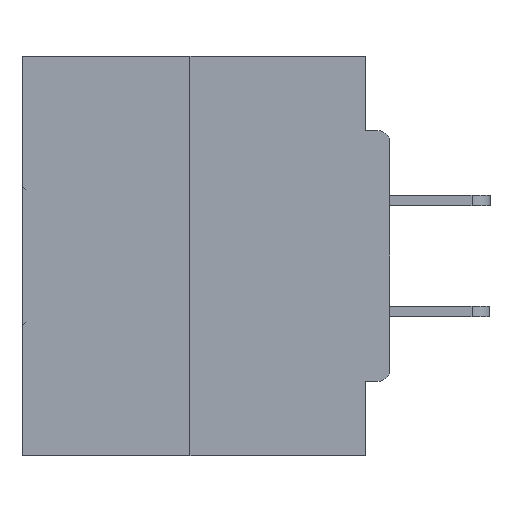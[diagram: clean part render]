
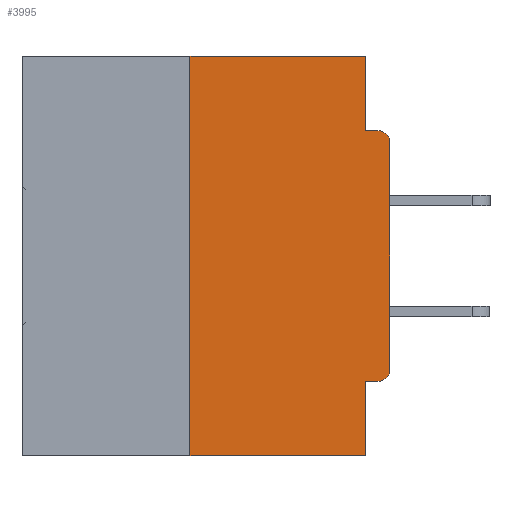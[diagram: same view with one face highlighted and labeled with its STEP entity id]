
A CAD part, left-side view. The second image highlights one B-rep face of the part: STEP entity #3995.
In plain terms, the highlighted planar face has unit normal (-1, 0, 0).
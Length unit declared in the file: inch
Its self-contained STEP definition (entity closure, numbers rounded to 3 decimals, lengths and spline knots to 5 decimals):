
#2 = CARTESIAN_POINT ( 'NONE',  ( 0., 0., -0.0935 ) ) ;
#969 = VERTEX_POINT ( 'NONE', #18899 ) ;
#1359 = CARTESIAN_POINT ( 'NONE',  ( 0., 0., -0.4065 ) ) ;
#1875 = ORIENTED_EDGE ( 'NONE', *, *, #18897, .F. ) ;
#2118 = AXIS2_PLACEMENT_3D ( 'NONE', #34022, #30119, #33000 ) ;
#2420 = EDGE_LOOP ( 'NONE', ( #34603, #5709, #41791, #29876, #35113, #34415, #11903, #22578, #1875, #41406 ) ) ;
#2688 = DIRECTION ( 'NONE',  ( 0., -1., 0. ) ) ;
#3995 = ADVANCED_FACE ( 'NONE', ( #31853 ), #4235, .F. ) ;
#4235 = PLANE ( 'NONE',  #2118 ) ;
#5149 = CARTESIAN_POINT ( 'NONE',  ( 0., 0., -0.1085 ) ) ;
#5591 = LINE ( 'NONE', #39703, #27346 ) ;
#5709 = ORIENTED_EDGE ( 'NONE', *, *, #39803, .F. ) ;
#6147 = DIRECTION ( 'NONE',  ( 0., -1., 0. ) ) ;
#6882 = DIRECTION ( 'NONE',  ( 0., 0., -1. ) ) ;
#8813 = EDGE_CURVE ( 'NONE', #32514, #969, #5591, .T. ) ;
#9744 = EDGE_CURVE ( 'NONE', #12409, #41118, #32910, .T. ) ;
#11856 = AXIS2_PLACEMENT_3D ( 'NONE', #23440, #13942, #36857 ) ;
#11903 = ORIENTED_EDGE ( 'NONE', *, *, #36400, .T. ) ;
#12409 = VERTEX_POINT ( 'NONE', #5149 ) ;
#13756 = DIRECTION ( 'NONE',  ( 0., -1., 0. ) ) ;
#13942 = DIRECTION ( 'NONE',  ( -1., 0., 0. ) ) ;
#14236 = DIRECTION ( 'NONE',  ( 0., 0., -1. ) ) ;
#14501 = LINE ( 'NONE', #20403, #20781 ) ;
#14518 = CARTESIAN_POINT ( 'NONE',  ( 0., 0.015, -0.3915 ) ) ;
#15038 = EDGE_CURVE ( 'NONE', #15554, #34817, #14501, .T. ) ;
#15059 = VERTEX_POINT ( 'NONE', #40153 ) ;
#15554 = VERTEX_POINT ( 'NONE', #39724 ) ;
#15796 = DIRECTION ( 'NONE',  ( 0., 0., 1. ) ) ;
#17372 = VECTOR ( 'NONE', #21396, 39.37008 ) ;
#17825 = CARTESIAN_POINT ( 'NONE',  ( 0., 0., 0. ) ) ;
#18897 = EDGE_CURVE ( 'NONE', #15059, #41118, #18935, .T. ) ;
#18899 = CARTESIAN_POINT ( 'NONE',  ( 0., 0.031, -0.5 ) ) ;
#18935 = LINE ( 'NONE', #2, #39032 ) ;
#19994 = VERTEX_POINT ( 'NONE', #35461 ) ;
#20403 = CARTESIAN_POINT ( 'NONE',  ( 0., 0.46, 0. ) ) ;
#20781 = VECTOR ( 'NONE', #13756, 39.37008 ) ;
#20797 = LINE ( 'NONE', #17825, #21312 ) ;
#21312 = VECTOR ( 'NONE', #30952, 39.37008 ) ;
#21396 = DIRECTION ( 'NONE',  ( 0., 1., 0. ) ) ;
#21541 = LINE ( 'NONE', #42221, #35944 ) ;
#22578 = ORIENTED_EDGE ( 'NONE', *, *, #9744, .T. ) ;
#22989 = CARTESIAN_POINT ( 'NONE',  ( 0., 0., -0.3915 ) ) ;
#23440 = CARTESIAN_POINT ( 'NONE',  ( 0., 0.015, -0.1085 ) ) ;
#23469 = VECTOR ( 'NONE', #6882, 39.37008 ) ;
#23548 = DIRECTION ( 'NONE',  ( 0., 0., -1. ) ) ;
#23867 = LINE ( 'NONE', #25965, #35254 ) ;
#25965 = CARTESIAN_POINT ( 'NONE',  ( 0., 0.46, -0.5 ) ) ;
#26995 = CARTESIAN_POINT ( 'NONE',  ( 0., 0.015, -0.4065 ) ) ;
#27091 = VERTEX_POINT ( 'NONE', #22989 ) ;
#27346 = VECTOR ( 'NONE', #23548, 39.37008 ) ;
#28159 = CARTESIAN_POINT ( 'NONE',  ( 0., 0.031, -0.4065 ) ) ;
#29846 = VERTEX_POINT ( 'NONE', #26995 ) ;
#29876 = ORIENTED_EDGE ( 'NONE', *, *, #8813, .F. ) ;
#29980 = EDGE_CURVE ( 'NONE', #29846, #32514, #41639, .T. ) ;
#30119 = DIRECTION ( 'NONE',  ( 1., 0., 0. ) ) ;
#30197 = CARTESIAN_POINT ( 'NONE',  ( 0., 0.015, -0.0935 ) ) ;
#30952 = DIRECTION ( 'NONE',  ( 0., 0., 1. ) ) ;
#31853 = FACE_OUTER_BOUND ( 'NONE', #2420, .T. ) ;
#32514 = VERTEX_POINT ( 'NONE', #28159 ) ;
#32828 = EDGE_CURVE ( 'NONE', #19994, #969, #23867, .T. ) ;
#32910 = CIRCLE ( 'NONE', #11856, 0.015 ) ;
#33000 = DIRECTION ( 'NONE',  ( 0., 0., -1. ) ) ;
#33824 = AXIS2_PLACEMENT_3D ( 'NONE', #14518, #34135, #14236 ) ;
#34001 = CIRCLE ( 'NONE', #33824, 0.015 ) ;
#34022 = CARTESIAN_POINT ( 'NONE',  ( 0., 0.46, 0. ) ) ;
#34135 = DIRECTION ( 'NONE',  ( -1., 0., 0. ) ) ;
#34415 = ORIENTED_EDGE ( 'NONE', *, *, #35000, .T. ) ;
#34603 = ORIENTED_EDGE ( 'NONE', *, *, #15038, .F. ) ;
#34817 = VERTEX_POINT ( 'NONE', #41098 ) ;
#35000 = EDGE_CURVE ( 'NONE', #29846, #27091, #34001, .T. ) ;
#35113 = ORIENTED_EDGE ( 'NONE', *, *, #29980, .F. ) ;
#35254 = VECTOR ( 'NONE', #6147, 39.37008 ) ;
#35461 = CARTESIAN_POINT ( 'NONE',  ( 0., 0.25, -0.5 ) ) ;
#35944 = VECTOR ( 'NONE', #15796, 39.37008 ) ;
#36400 = EDGE_CURVE ( 'NONE', #27091, #12409, #20797, .T. ) ;
#36857 = DIRECTION ( 'NONE',  ( 0., 0., -1. ) ) ;
#39032 = VECTOR ( 'NONE', #2688, 39.37008 ) ;
#39242 = CARTESIAN_POINT ( 'NONE',  ( 0., 0.031, 0. ) ) ;
#39703 = CARTESIAN_POINT ( 'NONE',  ( 0., 0.031, -0.5 ) ) ;
#39724 = CARTESIAN_POINT ( 'NONE',  ( 0., 0.25, 0. ) ) ;
#39803 = EDGE_CURVE ( 'NONE', #19994, #15554, #21541, .T. ) ;
#40153 = CARTESIAN_POINT ( 'NONE',  ( 0., 0.031, -0.0935 ) ) ;
#40444 = EDGE_CURVE ( 'NONE', #34817, #15059, #42585, .T. ) ;
#41098 = CARTESIAN_POINT ( 'NONE',  ( 0., 0.031, 0. ) ) ;
#41118 = VERTEX_POINT ( 'NONE', #30197 ) ;
#41406 = ORIENTED_EDGE ( 'NONE', *, *, #40444, .F. ) ;
#41639 = LINE ( 'NONE', #1359, #17372 ) ;
#41791 = ORIENTED_EDGE ( 'NONE', *, *, #32828, .T. ) ;
#42221 = CARTESIAN_POINT ( 'NONE',  ( 0., 0.25, 0. ) ) ;
#42585 = LINE ( 'NONE', #39242, #23469 ) ;
